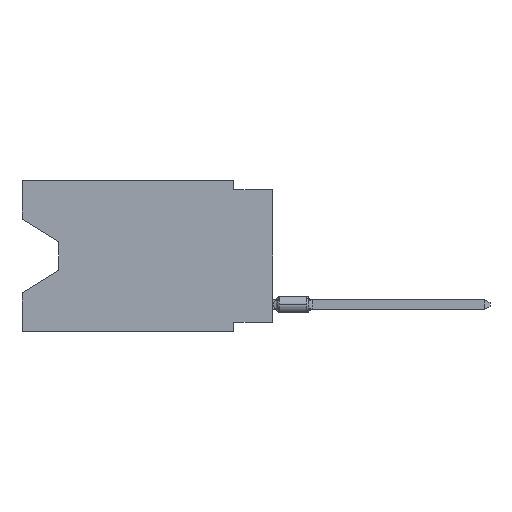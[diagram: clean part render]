
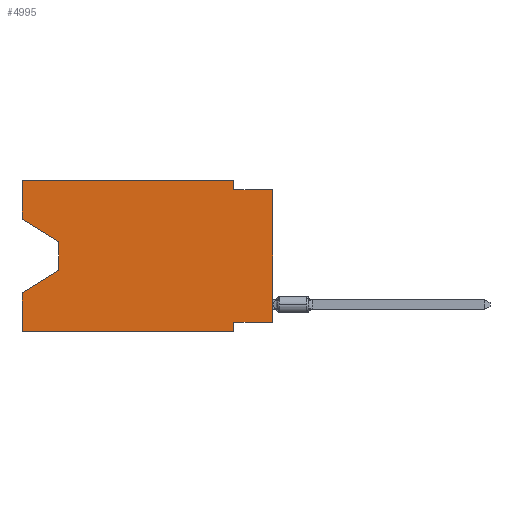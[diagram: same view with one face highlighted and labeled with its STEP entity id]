
A CAD part, left-side view. The second image highlights one B-rep face of the part: STEP entity #4995.
In plain terms, the highlighted planar face has unit normal (-1, 0, 0).
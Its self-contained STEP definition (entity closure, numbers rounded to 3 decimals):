
#276 = VERTEX_POINT ( 'NONE', #1760 ) ;
#353 = VERTEX_POINT ( 'NONE', #6092 ) ;
#489 = EDGE_CURVE ( 'NONE', #5042, #17123, #7601, .T. ) ;
#508 = CARTESIAN_POINT ( 'NONE',  ( 0., 13.97, -5.893 ) ) ;
#1411 = CARTESIAN_POINT ( 'NONE',  ( 0., 2.54, -9.906 ) ) ;
#1502 = VERTEX_POINT ( 'NONE', #14051 ) ;
#1760 = CARTESIAN_POINT ( 'NONE',  ( 0., 16.383, -2.546 ) ) ;
#1782 = ORIENTED_EDGE ( 'NONE', *, *, #23172, .F. ) ;
#2019 = VERTEX_POINT ( 'NONE', #8476 ) ;
#2020 = VECTOR ( 'NONE', #16806, 1000. ) ;
#2083 = ORIENTED_EDGE ( 'NONE', *, *, #17317, .F. ) ;
#2445 = AXIS2_PLACEMENT_3D ( 'NONE', #21158, #4671, #2872 ) ;
#2740 = CARTESIAN_POINT ( 'NONE',  ( 0., 16.383, -2.546 ) ) ;
#2747 = PLANE ( 'NONE',  #2445 ) ;
#2872 = DIRECTION ( 'NONE',  ( 0., 0., -1. ) ) ;
#3116 = DIRECTION ( 'NONE',  ( 0., 0., 1. ) ) ;
#3576 = VECTOR ( 'NONE', #11332, 1000. ) ;
#3578 = CARTESIAN_POINT ( 'NONE',  ( 0., 13.97, -4.013 ) ) ;
#3802 = VERTEX_POINT ( 'NONE', #22379 ) ;
#3909 = VECTOR ( 'NONE', #10545, 1000. ) ;
#4671 = DIRECTION ( 'NONE',  ( 1., 0., 0. ) ) ;
#4702 = ORIENTED_EDGE ( 'NONE', *, *, #12671, .F. ) ;
#4838 = ORIENTED_EDGE ( 'NONE', *, *, #23098, .T. ) ;
#4995 = ADVANCED_FACE ( 'NONE', ( #12492 ), #2747, .F. ) ;
#5031 = CARTESIAN_POINT ( 'NONE',  ( 0., 0., -0.635 ) ) ;
#5042 = VERTEX_POINT ( 'NONE', #3578 ) ;
#5181 = CARTESIAN_POINT ( 'NONE',  ( 0., 16.383, 0. ) ) ;
#5633 = CARTESIAN_POINT ( 'NONE',  ( 0., 2.54, -9.271 ) ) ;
#5726 = CARTESIAN_POINT ( 'NONE',  ( 0., 16.383, 0. ) ) ;
#5930 = LINE ( 'NONE', #9411, #3576 ) ;
#6092 = CARTESIAN_POINT ( 'NONE',  ( 0., 16.383, -9.906 ) ) ;
#6136 = VERTEX_POINT ( 'NONE', #5031 ) ;
#6601 = VECTOR ( 'NONE', #3116, 1000. ) ;
#7591 = VERTEX_POINT ( 'NONE', #12080 ) ;
#7601 = LINE ( 'NONE', #18310, #12290 ) ;
#8008 = LINE ( 'NONE', #15341, #8700 ) ;
#8175 = VECTOR ( 'NONE', #19228, 1000. ) ;
#8476 = CARTESIAN_POINT ( 'NONE',  ( 0., 16.383, -7.36 ) ) ;
#8689 = EDGE_CURVE ( 'NONE', #17123, #2019, #8008, .T. ) ;
#8700 = VECTOR ( 'NONE', #22678, 1000. ) ;
#8831 = CARTESIAN_POINT ( 'NONE',  ( 0., 0., 0. ) ) ;
#9206 = ORIENTED_EDGE ( 'NONE', *, *, #23585, .F. ) ;
#9411 = CARTESIAN_POINT ( 'NONE',  ( 0., 2.54, 0. ) ) ;
#9451 = VERTEX_POINT ( 'NONE', #15378 ) ;
#10545 = DIRECTION ( 'NONE',  ( 0., -1., 0. ) ) ;
#10642 = EDGE_LOOP ( 'NONE', ( #14127, #17383, #15709, #2083, #15001, #4702, #1782, #4838, #18841, #11766, #19061, #9206 ) ) ;
#10645 = DIRECTION ( 'NONE',  ( 0., 0., 1. ) ) ;
#10804 = LINE ( 'NONE', #5726, #2020 ) ;
#10893 = LINE ( 'NONE', #19788, #3909 ) ;
#10987 = LINE ( 'NONE', #8831, #13214 ) ;
#11332 = DIRECTION ( 'NONE',  ( 0., 0., -1. ) ) ;
#11766 = ORIENTED_EDGE ( 'NONE', *, *, #18271, .F. ) ;
#11933 = EDGE_CURVE ( 'NONE', #7591, #6136, #23092, .T. ) ;
#12080 = CARTESIAN_POINT ( 'NONE',  ( 0., 2.54, -0.635 ) ) ;
#12290 = VECTOR ( 'NONE', #22403, 1000. ) ;
#12492 = FACE_OUTER_BOUND ( 'NONE', #10642, .T. ) ;
#12671 = EDGE_CURVE ( 'NONE', #22334, #9451, #23304, .T. ) ;
#13214 = VECTOR ( 'NONE', #10645, 1000. ) ;
#13254 = LINE ( 'NONE', #16969, #18094 ) ;
#13464 = LINE ( 'NONE', #2740, #8175 ) ;
#13712 = EDGE_CURVE ( 'NONE', #276, #5042, #13464, .T. ) ;
#13730 = DIRECTION ( 'NONE',  ( 0., -1., 0. ) ) ;
#13967 = LINE ( 'NONE', #5181, #6601 ) ;
#14051 = CARTESIAN_POINT ( 'NONE',  ( 0., 2.54, 0. ) ) ;
#14101 = EDGE_CURVE ( 'NONE', #14806, #1502, #10804, .T. ) ;
#14127 = ORIENTED_EDGE ( 'NONE', *, *, #13712, .T. ) ;
#14208 = VECTOR ( 'NONE', #13730, 1000. ) ;
#14238 = DIRECTION ( 'NONE',  ( 0., 1., 0. ) ) ;
#14241 = VECTOR ( 'NONE', #15727, 1000. ) ;
#14721 = VECTOR ( 'NONE', #14238, 1000. ) ;
#14806 = VERTEX_POINT ( 'NONE', #18070 ) ;
#15001 = ORIENTED_EDGE ( 'NONE', *, *, #17757, .T. ) ;
#15341 = CARTESIAN_POINT ( 'NONE',  ( 0., 13.97, -5.893 ) ) ;
#15378 = CARTESIAN_POINT ( 'NONE',  ( 0., 2.54, -9.906 ) ) ;
#15644 = CARTESIAN_POINT ( 'NONE',  ( 0., 0., -0.635 ) ) ;
#15709 = ORIENTED_EDGE ( 'NONE', *, *, #8689, .T. ) ;
#15727 = DIRECTION ( 'NONE',  ( 0., 0., -1. ) ) ;
#16054 = CARTESIAN_POINT ( 'NONE',  ( 0., 0., -9.271 ) ) ;
#16514 = LINE ( 'NONE', #16054, #14721 ) ;
#16806 = DIRECTION ( 'NONE',  ( 0., -1., 0. ) ) ;
#16969 = CARTESIAN_POINT ( 'NONE',  ( 0., 16.383, 0. ) ) ;
#17123 = VERTEX_POINT ( 'NONE', #508 ) ;
#17317 = EDGE_CURVE ( 'NONE', #353, #2019, #13967, .T. ) ;
#17383 = ORIENTED_EDGE ( 'NONE', *, *, #489, .T. ) ;
#17757 = EDGE_CURVE ( 'NONE', #353, #9451, #10893, .T. ) ;
#18070 = CARTESIAN_POINT ( 'NONE',  ( 0., 16.383, 0. ) ) ;
#18094 = VECTOR ( 'NONE', #20212, 1000. ) ;
#18271 = EDGE_CURVE ( 'NONE', #1502, #7591, #5930, .T. ) ;
#18310 = CARTESIAN_POINT ( 'NONE',  ( 0., 13.97, -4.013 ) ) ;
#18841 = ORIENTED_EDGE ( 'NONE', *, *, #11933, .F. ) ;
#19061 = ORIENTED_EDGE ( 'NONE', *, *, #14101, .F. ) ;
#19228 = DIRECTION ( 'NONE',  ( 0., -0.855, -0.519 ) ) ;
#19788 = CARTESIAN_POINT ( 'NONE',  ( 0., 16.383, -9.906 ) ) ;
#20212 = DIRECTION ( 'NONE',  ( 0., 0., 1. ) ) ;
#21158 = CARTESIAN_POINT ( 'NONE',  ( 0., 16.383, 0. ) ) ;
#22334 = VERTEX_POINT ( 'NONE', #5633 ) ;
#22379 = CARTESIAN_POINT ( 'NONE',  ( 0., 0., -9.271 ) ) ;
#22403 = DIRECTION ( 'NONE',  ( 0., 0., -1. ) ) ;
#22678 = DIRECTION ( 'NONE',  ( 0., 0.855, -0.519 ) ) ;
#23092 = LINE ( 'NONE', #15644, #14208 ) ;
#23098 = EDGE_CURVE ( 'NONE', #3802, #6136, #10987, .T. ) ;
#23172 = EDGE_CURVE ( 'NONE', #3802, #22334, #16514, .T. ) ;
#23304 = LINE ( 'NONE', #1411, #14241 ) ;
#23585 = EDGE_CURVE ( 'NONE', #276, #14806, #13254, .T. ) ;
